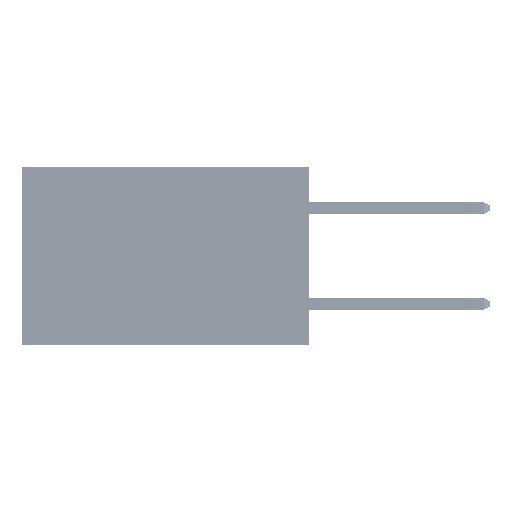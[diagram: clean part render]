
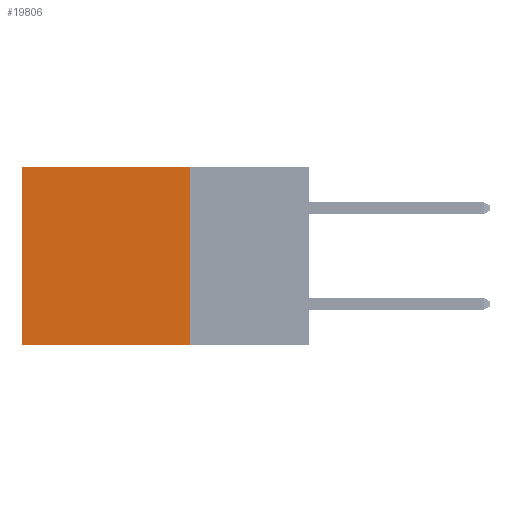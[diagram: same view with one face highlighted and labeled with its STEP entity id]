
A CAD part, left-side view. The second image highlights one B-rep face of the part: STEP entity #19806.
In plain terms, the highlighted planar face has unit normal (-1, 0, 0).
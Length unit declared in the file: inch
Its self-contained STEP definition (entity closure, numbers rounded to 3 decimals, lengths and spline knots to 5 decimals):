
#77 = LINE ( 'NONE', #12957, #6805 ) ;
#4999 = EDGE_CURVE ( 'NONE', #46425, #8027, #38981, .T. ) ;
#5715 = DIRECTION ( 'NONE',  ( 0., 1., 0. ) ) ;
#6805 = VECTOR ( 'NONE', #8926, 39.37008 ) ;
#8027 = VERTEX_POINT ( 'NONE', #9282 ) ;
#8672 = ORIENTED_EDGE ( 'NONE', *, *, #4999, .T. ) ;
#8926 = DIRECTION ( 'NONE',  ( 0., 0., -1. ) ) ;
#9282 = CARTESIAN_POINT ( 'NONE',  ( 0.2875, 0.6, -0.37 ) ) ;
#10775 = EDGE_CURVE ( 'NONE', #48045, #8027, #20047, .T. ) ;
#11431 = DIRECTION ( 'NONE',  ( 0., 1., 0. ) ) ;
#11953 = PLANE ( 'NONE',  #33079 ) ;
#12957 = CARTESIAN_POINT ( 'NONE',  ( 0.2875, 0.25, 0. ) ) ;
#14617 = DIRECTION ( 'NONE',  ( 0., 0., -1. ) ) ;
#18732 = VECTOR ( 'NONE', #5715, 39.37008 ) ;
#19806 = ADVANCED_FACE ( 'NONE', ( #43827 ), #11953, .F. ) ;
#20047 = LINE ( 'NONE', #36326, #43642 ) ;
#21076 = EDGE_LOOP ( 'NONE', ( #8672, #21912, #23325, #46326 ) ) ;
#21912 = ORIENTED_EDGE ( 'NONE', *, *, #10775, .F. ) ;
#22092 = CARTESIAN_POINT ( 'NONE',  ( 0.2875, 0.25, 0. ) ) ;
#22362 = LINE ( 'NONE', #22092, #18732 ) ;
#22904 = VERTEX_POINT ( 'NONE', #42694 ) ;
#23325 = ORIENTED_EDGE ( 'NONE', *, *, #45330, .F. ) ;
#25899 = EDGE_CURVE ( 'NONE', #22904, #46425, #22362, .T. ) ;
#27253 = CARTESIAN_POINT ( 'NONE',  ( 0.2875, 0.25, 0. ) ) ;
#28052 = DIRECTION ( 'NONE',  ( 1., 0., 0. ) ) ;
#30744 = CARTESIAN_POINT ( 'NONE',  ( 0.2875, 0.6, 0. ) ) ;
#32357 = VECTOR ( 'NONE', #14617, 39.37008 ) ;
#33079 = AXIS2_PLACEMENT_3D ( 'NONE', #27253, #28052, #52657 ) ;
#36326 = CARTESIAN_POINT ( 'NONE',  ( 0.2875, 0.25, -0.37 ) ) ;
#37983 = CARTESIAN_POINT ( 'NONE',  ( 0.2875, 0.6, 0. ) ) ;
#38981 = LINE ( 'NONE', #37983, #32357 ) ;
#42694 = CARTESIAN_POINT ( 'NONE',  ( 0.2875, 0.25, 0. ) ) ;
#43642 = VECTOR ( 'NONE', #11431, 39.37008 ) ;
#43827 = FACE_OUTER_BOUND ( 'NONE', #21076, .T. ) ;
#44889 = CARTESIAN_POINT ( 'NONE',  ( 0.2875, 0.25, -0.37 ) ) ;
#45330 = EDGE_CURVE ( 'NONE', #22904, #48045, #77, .T. ) ;
#46326 = ORIENTED_EDGE ( 'NONE', *, *, #25899, .T. ) ;
#46425 = VERTEX_POINT ( 'NONE', #30744 ) ;
#48045 = VERTEX_POINT ( 'NONE', #44889 ) ;
#52657 = DIRECTION ( 'NONE',  ( 0., 0., -1. ) ) ;
